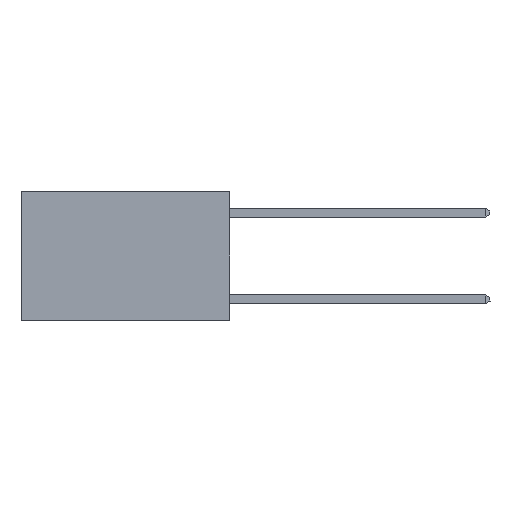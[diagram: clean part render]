
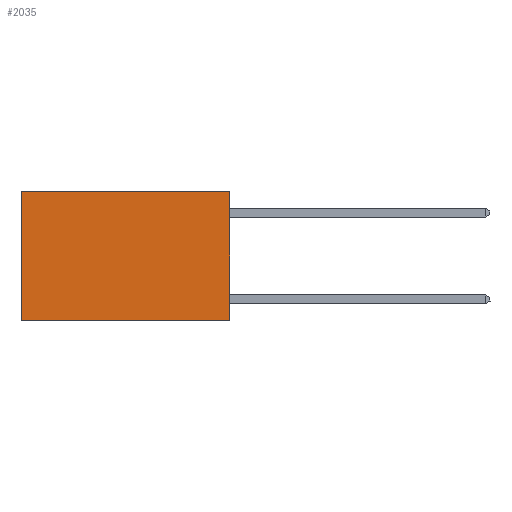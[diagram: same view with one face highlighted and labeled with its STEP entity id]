
A CAD part, left-side view. The second image highlights one B-rep face of the part: STEP entity #2035.
In plain terms, the highlighted planar face has unit normal (-1, 0, 0).
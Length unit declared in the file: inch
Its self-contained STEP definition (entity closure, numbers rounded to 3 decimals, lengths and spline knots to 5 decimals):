
#342 = EDGE_CURVE ( 'NONE', #18917, #6941, #8412, .T. ) ;
#617 = ORIENTED_EDGE ( 'NONE', *, *, #14883, .F. ) ;
#718 = AXIS2_PLACEMENT_3D ( 'NONE', #16271, #11415, #1673 ) ;
#1618 = DIRECTION ( 'NONE',  ( 0., 1., 0. ) ) ;
#1673 = DIRECTION ( 'NONE',  ( 0., 0., -1. ) ) ;
#1725 = LINE ( 'NONE', #13676, #14204 ) ;
#2035 = ADVANCED_FACE ( 'NONE', ( #20725 ), #3238, .F. ) ;
#2510 = ORIENTED_EDGE ( 'NONE', *, *, #5396, .T. ) ;
#2672 = LINE ( 'NONE', #16431, #7022 ) ;
#3238 = PLANE ( 'NONE',  #718 ) ;
#3530 = DIRECTION ( 'NONE',  ( 0., 0., -1. ) ) ;
#4107 = VECTOR ( 'NONE', #18497, 39.37008 ) ;
#5396 = EDGE_CURVE ( 'NONE', #18938, #18917, #2672, .T. ) ;
#6941 = VERTEX_POINT ( 'NONE', #9120 ) ;
#7022 = VECTOR ( 'NONE', #18017, 39.37008 ) ;
#7030 = CARTESIAN_POINT ( 'NONE',  ( 0.2625, 0.6, 0. ) ) ;
#7230 = ORIENTED_EDGE ( 'NONE', *, *, #12912, .F. ) ;
#7632 = LINE ( 'NONE', #11648, #15296 ) ;
#8412 = LINE ( 'NONE', #15459, #4107 ) ;
#9120 = CARTESIAN_POINT ( 'NONE',  ( 0.2625, 0.6, -0.37 ) ) ;
#11068 = ORIENTED_EDGE ( 'NONE', *, *, #342, .T. ) ;
#11415 = DIRECTION ( 'NONE',  ( 1., 0., 0. ) ) ;
#11429 = CARTESIAN_POINT ( 'NONE',  ( 0.2625, 0., -0.37 ) ) ;
#11648 = CARTESIAN_POINT ( 'NONE',  ( 0.2625, 0., 0. ) ) ;
#12912 = EDGE_CURVE ( 'NONE', #18938, #18719, #7632, .T. ) ;
#13676 = CARTESIAN_POINT ( 'NONE',  ( 0.2625, 0., -0.37 ) ) ;
#14204 = VECTOR ( 'NONE', #1618, 39.37008 ) ;
#14883 = EDGE_CURVE ( 'NONE', #18719, #6941, #1725, .T. ) ;
#15296 = VECTOR ( 'NONE', #3530, 39.37008 ) ;
#15459 = CARTESIAN_POINT ( 'NONE',  ( 0.2625, 0.6, 0. ) ) ;
#16271 = CARTESIAN_POINT ( 'NONE',  ( 0.2625, 0., 0. ) ) ;
#16431 = CARTESIAN_POINT ( 'NONE',  ( 0.2625, 0., 0. ) ) ;
#16826 = CARTESIAN_POINT ( 'NONE',  ( 0.2625, 0., 0. ) ) ;
#18017 = DIRECTION ( 'NONE',  ( 0., 1., 0. ) ) ;
#18210 = EDGE_LOOP ( 'NONE', ( #11068, #617, #7230, #2510 ) ) ;
#18497 = DIRECTION ( 'NONE',  ( 0., 0., -1. ) ) ;
#18719 = VERTEX_POINT ( 'NONE', #11429 ) ;
#18917 = VERTEX_POINT ( 'NONE', #7030 ) ;
#18938 = VERTEX_POINT ( 'NONE', #16826 ) ;
#20725 = FACE_OUTER_BOUND ( 'NONE', #18210, .T. ) ;
